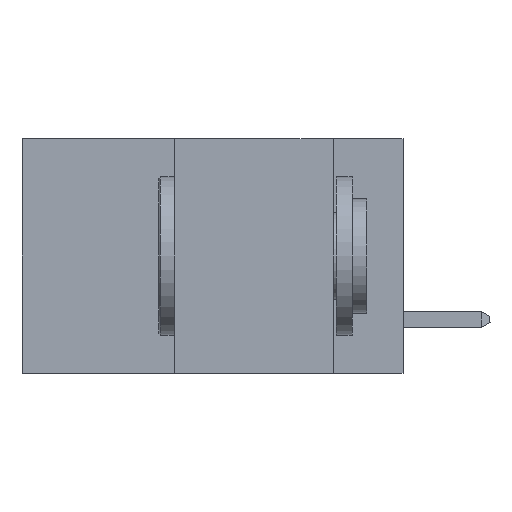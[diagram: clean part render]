
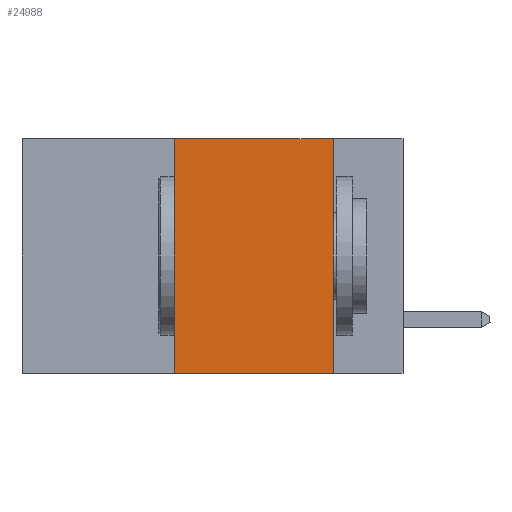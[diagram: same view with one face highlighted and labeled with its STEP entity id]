
A CAD part, left-side view. The second image highlights one B-rep face of the part: STEP entity #24988.
In plain terms, the highlighted planar face has unit normal (-1, 0, 0).
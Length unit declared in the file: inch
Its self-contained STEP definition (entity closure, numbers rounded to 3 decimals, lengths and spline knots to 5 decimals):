
#843 = ORIENTED_EDGE ( 'NONE', *, *, #16529, .F. ) ;
#1275 = DIRECTION ( 'NONE',  ( 0., 0., -1. ) ) ;
#2230 = VECTOR ( 'NONE', #8689, 39.37008 ) ;
#2680 = FACE_OUTER_BOUND ( 'NONE', #33299, .T. ) ;
#3447 = CARTESIAN_POINT ( 'NONE',  ( 0., 0.11, -0.37 ) ) ;
#3935 = VERTEX_POINT ( 'NONE', #3447 ) ;
#6846 = CARTESIAN_POINT ( 'NONE',  ( 0., 0.36, -0.37 ) ) ;
#7132 = ORIENTED_EDGE ( 'NONE', *, *, #12805, .F. ) ;
#8689 = DIRECTION ( 'NONE',  ( 0., 0., -1. ) ) ;
#9083 = EDGE_CURVE ( 'NONE', #20555, #11845, #29439, .T. ) ;
#11670 = CARTESIAN_POINT ( 'NONE',  ( 0., 0.36, 0. ) ) ;
#11845 = VERTEX_POINT ( 'NONE', #22527 ) ;
#12275 = VECTOR ( 'NONE', #26818, 39.37008 ) ;
#12386 = VECTOR ( 'NONE', #22400, 39.37008 ) ;
#12805 = EDGE_CURVE ( 'NONE', #14612, #20555, #26202, .T. ) ;
#13564 = DIRECTION ( 'NONE',  ( 0., -1., 0. ) ) ;
#14612 = VERTEX_POINT ( 'NONE', #6846 ) ;
#15389 = PLANE ( 'NONE',  #28586 ) ;
#16355 = ORIENTED_EDGE ( 'NONE', *, *, #20988, .T. ) ;
#16529 = EDGE_CURVE ( 'NONE', #11845, #3935, #23777, .T. ) ;
#18190 = DIRECTION ( 'NONE',  ( 1., 0., 0. ) ) ;
#19115 = CARTESIAN_POINT ( 'NONE',  ( 0., 0.6, -0.37 ) ) ;
#19815 = LINE ( 'NONE', #19115, #12386 ) ;
#20555 = VERTEX_POINT ( 'NONE', #11670 ) ;
#20988 = EDGE_CURVE ( 'NONE', #14612, #3935, #19815, .T. ) ;
#21863 = CARTESIAN_POINT ( 'NONE',  ( 0., 0.6, 0. ) ) ;
#22176 = VECTOR ( 'NONE', #13564, 39.37008 ) ;
#22400 = DIRECTION ( 'NONE',  ( 0., -1., 0. ) ) ;
#22527 = CARTESIAN_POINT ( 'NONE',  ( 0., 0.11, 0. ) ) ;
#23777 = LINE ( 'NONE', #25385, #2230 ) ;
#24988 = ADVANCED_FACE ( 'NONE', ( #2680 ), #15389, .F. ) ;
#25385 = CARTESIAN_POINT ( 'NONE',  ( 0., 0.11, 0. ) ) ;
#26202 = LINE ( 'NONE', #29530, #12275 ) ;
#26432 = CARTESIAN_POINT ( 'NONE',  ( 0., 0.6, 0. ) ) ;
#26818 = DIRECTION ( 'NONE',  ( 0., 0., 1. ) ) ;
#28586 = AXIS2_PLACEMENT_3D ( 'NONE', #26432, #18190, #1275 ) ;
#29439 = LINE ( 'NONE', #21863, #22176 ) ;
#29530 = CARTESIAN_POINT ( 'NONE',  ( 0., 0.36, 0. ) ) ;
#31425 = ORIENTED_EDGE ( 'NONE', *, *, #9083, .F. ) ;
#33299 = EDGE_LOOP ( 'NONE', ( #843, #31425, #7132, #16355 ) ) ;
